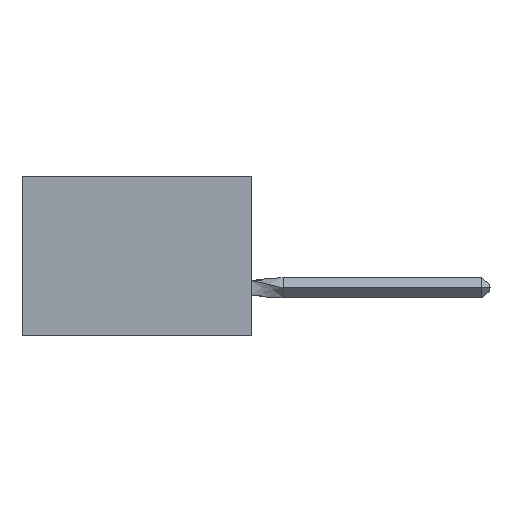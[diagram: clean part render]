
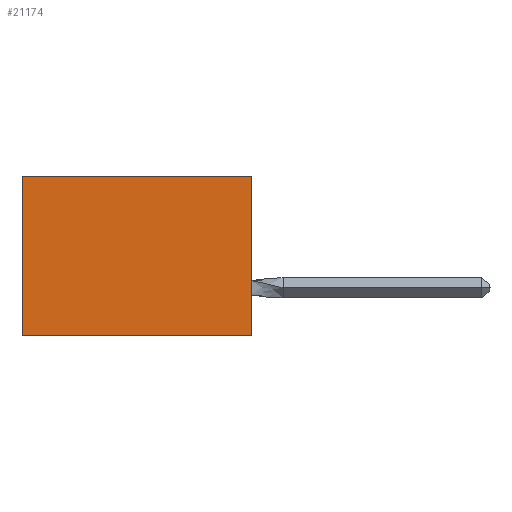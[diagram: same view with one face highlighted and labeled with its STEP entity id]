
A CAD part, left-side view. The second image highlights one B-rep face of the part: STEP entity #21174.
In plain terms, the highlighted planar face has unit normal (-1, 0, 0).
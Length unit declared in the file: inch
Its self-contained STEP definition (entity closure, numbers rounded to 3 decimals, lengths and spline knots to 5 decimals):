
#1288 = CARTESIAN_POINT ( 'NONE',  ( 0.305, 0., 0. ) ) ;
#4411 = ORIENTED_EDGE ( 'NONE', *, *, #32950, .F. ) ;
#4742 = VECTOR ( 'NONE', #14301, 39.37008 ) ;
#5193 = VECTOR ( 'NONE', #26379, 39.37008 ) ;
#7280 = CARTESIAN_POINT ( 'NONE',  ( 0.305, 0.72, -0.5 ) ) ;
#8912 = VECTOR ( 'NONE', #10352, 39.37008 ) ;
#10352 = DIRECTION ( 'NONE',  ( 0., 0., -1. ) ) ;
#11146 = ORIENTED_EDGE ( 'NONE', *, *, #37926, .T. ) ;
#12600 = VERTEX_POINT ( 'NONE', #35699 ) ;
#13214 = CARTESIAN_POINT ( 'NONE',  ( 0.305, 0., 0. ) ) ;
#13719 = CARTESIAN_POINT ( 'NONE',  ( 0.305, 0.72, 0. ) ) ;
#14301 = DIRECTION ( 'NONE',  ( 0., 0., -1. ) ) ;
#14314 = VERTEX_POINT ( 'NONE', #13719 ) ;
#16877 = VERTEX_POINT ( 'NONE', #13214 ) ;
#16970 = AXIS2_PLACEMENT_3D ( 'NONE', #20168, #18795, #29285 ) ;
#18795 = DIRECTION ( 'NONE',  ( 1., 0., 0. ) ) ;
#19570 = ORIENTED_EDGE ( 'NONE', *, *, #33365, .T. ) ;
#20035 = FACE_OUTER_BOUND ( 'NONE', #41342, .T. ) ;
#20168 = CARTESIAN_POINT ( 'NONE',  ( 0.305, 0., -0.5 ) ) ;
#20886 = VERTEX_POINT ( 'NONE', #35160 ) ;
#21174 = ADVANCED_FACE ( 'NONE', ( #20035 ), #32220, .F. ) ;
#26092 = CARTESIAN_POINT ( 'NONE',  ( 0.305, 0., -0.5 ) ) ;
#26379 = DIRECTION ( 'NONE',  ( 0., 1., 0. ) ) ;
#28669 = LINE ( 'NONE', #38314, #4742 ) ;
#29285 = DIRECTION ( 'NONE',  ( 0., 0., -1. ) ) ;
#31258 = LINE ( 'NONE', #26092, #5193 ) ;
#32220 = PLANE ( 'NONE',  #16970 ) ;
#32950 = EDGE_CURVE ( 'NONE', #12600, #20886, #31258, .T. ) ;
#33365 = EDGE_CURVE ( 'NONE', #16877, #14314, #36166, .T. ) ;
#35160 = CARTESIAN_POINT ( 'NONE',  ( 0.305, 0.72, -0.5 ) ) ;
#35699 = CARTESIAN_POINT ( 'NONE',  ( 0.305, 0., -0.5 ) ) ;
#36108 = DIRECTION ( 'NONE',  ( 0., 1., 0. ) ) ;
#36166 = LINE ( 'NONE', #1288, #38894 ) ;
#37926 = EDGE_CURVE ( 'NONE', #14314, #20886, #44368, .T. ) ;
#38314 = CARTESIAN_POINT ( 'NONE',  ( 0.305, 0., -0.5 ) ) ;
#38716 = ORIENTED_EDGE ( 'NONE', *, *, #41051, .F. ) ;
#38894 = VECTOR ( 'NONE', #36108, 39.37008 ) ;
#41051 = EDGE_CURVE ( 'NONE', #16877, #12600, #28669, .T. ) ;
#41342 = EDGE_LOOP ( 'NONE', ( #11146, #4411, #38716, #19570 ) ) ;
#44368 = LINE ( 'NONE', #7280, #8912 ) ;
